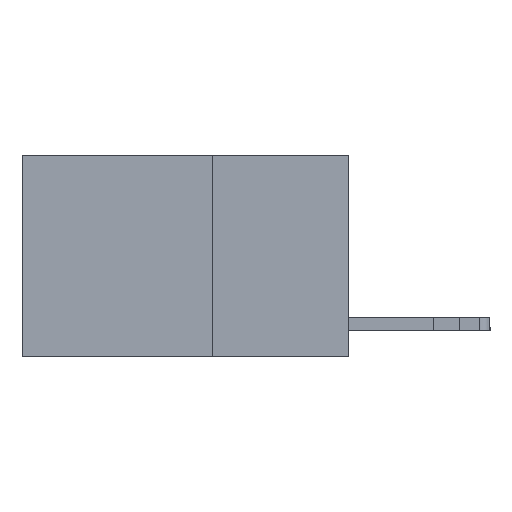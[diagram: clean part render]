
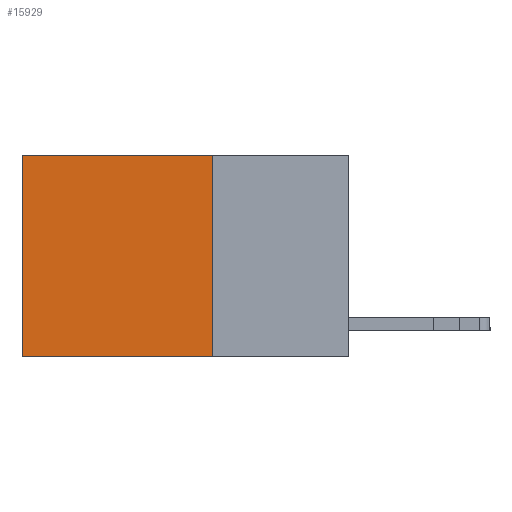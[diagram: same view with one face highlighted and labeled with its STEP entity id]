
A CAD part, left-side view. The second image highlights one B-rep face of the part: STEP entity #15929.
In plain terms, the highlighted planar face has unit normal (-1, 0, 0).
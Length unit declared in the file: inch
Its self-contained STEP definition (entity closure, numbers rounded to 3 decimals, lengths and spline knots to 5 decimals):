
#688 = LINE ( 'NONE', #3260, #7799 ) ;
#1300 = EDGE_CURVE ( 'NONE', #17206, #14619, #17362, .T. ) ;
#1864 = EDGE_CURVE ( 'NONE', #13225, #14619, #4902, .T. ) ;
#2141 = VECTOR ( 'NONE', #2150, 39.37008 ) ;
#2150 = DIRECTION ( 'NONE',  ( 0., 1., 0. ) ) ;
#2444 = DIRECTION ( 'NONE',  ( 1., 0., 0. ) ) ;
#3241 = ORIENTED_EDGE ( 'NONE', *, *, #1300, .T. ) ;
#3260 = CARTESIAN_POINT ( 'NONE',  ( 0.2625, 0.25, 0. ) ) ;
#3589 = VECTOR ( 'NONE', #4588, 39.37008 ) ;
#3769 = EDGE_CURVE ( 'NONE', #5720, #13225, #688, .T. ) ;
#4588 = DIRECTION ( 'NONE',  ( 0., 1., 0. ) ) ;
#4902 = LINE ( 'NONE', #6190, #2141 ) ;
#5720 = VERTEX_POINT ( 'NONE', #7089 ) ;
#6190 = CARTESIAN_POINT ( 'NONE',  ( 0.2625, 0.25, -0.37 ) ) ;
#6643 = CARTESIAN_POINT ( 'NONE',  ( 0.2625, 0.6, -0.37 ) ) ;
#7089 = CARTESIAN_POINT ( 'NONE',  ( 0.2625, 0.25, 0. ) ) ;
#7708 = LINE ( 'NONE', #14727, #3589 ) ;
#7799 = VECTOR ( 'NONE', #11911, 39.37008 ) ;
#7955 = PLANE ( 'NONE',  #12198 ) ;
#8425 = ORIENTED_EDGE ( 'NONE', *, *, #9287, .T. ) ;
#9215 = CARTESIAN_POINT ( 'NONE',  ( 0.2625, 0.25, -0.37 ) ) ;
#9287 = EDGE_CURVE ( 'NONE', #5720, #17206, #7708, .T. ) ;
#10558 = EDGE_LOOP ( 'NONE', ( #3241, #14278, #12576, #8425 ) ) ;
#11911 = DIRECTION ( 'NONE',  ( 0., 0., -1. ) ) ;
#12104 = FACE_OUTER_BOUND ( 'NONE', #10558, .T. ) ;
#12198 = AXIS2_PLACEMENT_3D ( 'NONE', #17678, #2444, #17952 ) ;
#12576 = ORIENTED_EDGE ( 'NONE', *, *, #3769, .F. ) ;
#12604 = CARTESIAN_POINT ( 'NONE',  ( 0.2625, 0.6, 0. ) ) ;
#13225 = VERTEX_POINT ( 'NONE', #9215 ) ;
#14278 = ORIENTED_EDGE ( 'NONE', *, *, #1864, .F. ) ;
#14469 = CARTESIAN_POINT ( 'NONE',  ( 0.2625, 0.6, 0. ) ) ;
#14619 = VERTEX_POINT ( 'NONE', #6643 ) ;
#14727 = CARTESIAN_POINT ( 'NONE',  ( 0.2625, 0.25, 0. ) ) ;
#15929 = ADVANCED_FACE ( 'NONE', ( #12104 ), #7955, .F. ) ;
#17206 = VERTEX_POINT ( 'NONE', #12604 ) ;
#17362 = LINE ( 'NONE', #14469, #17451 ) ;
#17451 = VECTOR ( 'NONE', #17550, 39.37008 ) ;
#17550 = DIRECTION ( 'NONE',  ( 0., 0., -1. ) ) ;
#17678 = CARTESIAN_POINT ( 'NONE',  ( 0.2625, 0.25, 0. ) ) ;
#17952 = DIRECTION ( 'NONE',  ( 0., 0., -1. ) ) ;
